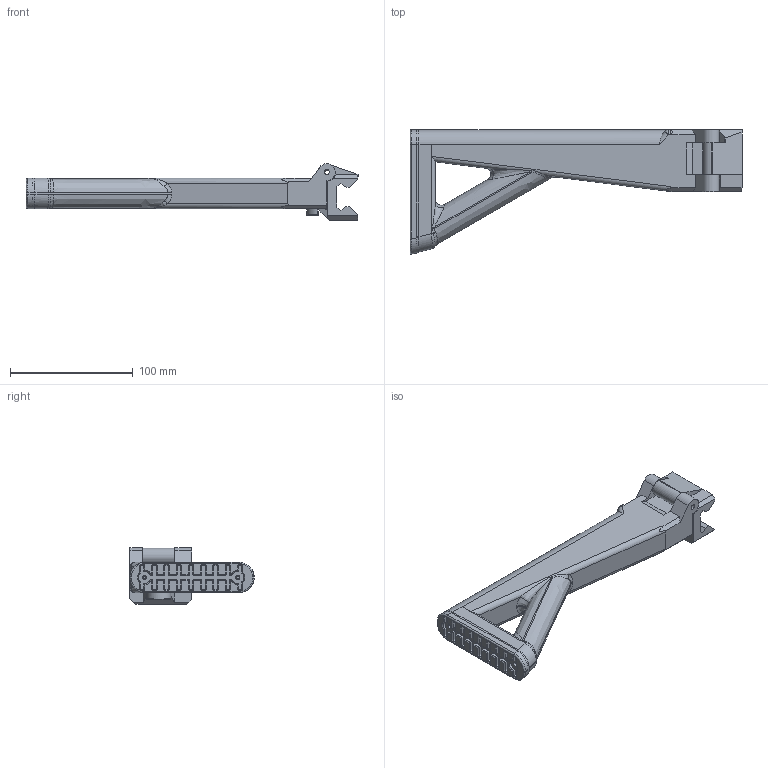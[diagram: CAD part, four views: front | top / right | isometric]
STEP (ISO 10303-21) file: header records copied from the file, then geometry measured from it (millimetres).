
FILE_DESCRIPTION(/* description */ (''),/* implementation_level */ '2;1');
FILE_NAME(/* author */ (''),/* organization */ (''),/* preprocessor_version */ 'ST-DEVELOPER v15.2',/* originating_system */ 'Autodesk Translator Framework v2.0.0.5431',/* authorisation */ '');
FILE_SCHEMA (('AUTOMOTIVE_DESIGN { 1 0 10303 214 3 1 1 }'));
Length unit declared in the file: centimetre
Products named in the file (1): unpublished stocks
Bounding box: 270.92 x 101.42 x 46.3 mm (x, y, z)
Volume: 334805.3 mm3; surface area: 64511.5 mm2
Topology: 4 solids, 4 shells, 556 faces, 1388 edges, 843 vertices
Faces by surface type: plane 261, cylinder 153, cone 73, bspline 30, torus 21, sphere 18
Full cylindrical faces by diameter (mm): 2.5 x2, 3 x1, 3.5 x2, 4 x3, 12.1 x1, 20.5 x1
Entity records: 17626 total; most frequent: CARTESIAN_POINT 4400, DIRECTION 2780, ORIENTED_EDGE 2742, EDGE_CURVE 1371, AXIS2_PLACEMENT_3D 969, LINE 842, VECTOR 842, VERTEX_POINT 838
